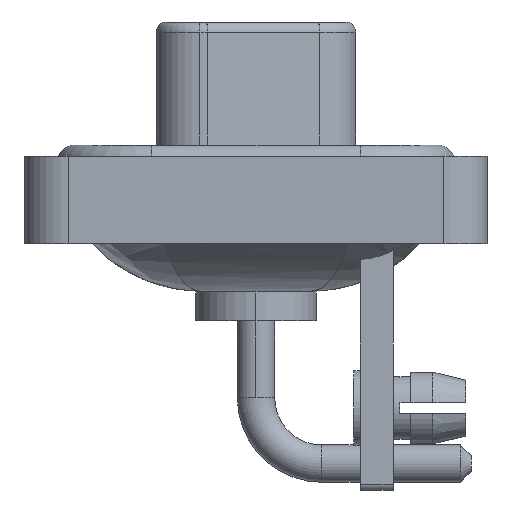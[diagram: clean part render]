
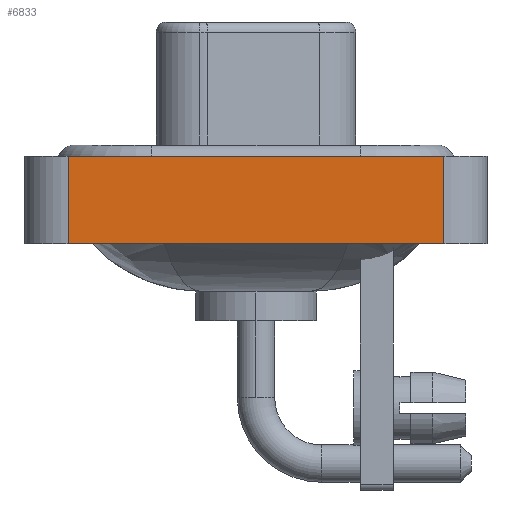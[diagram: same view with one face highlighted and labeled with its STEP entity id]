
A CAD part, left-side view. The second image highlights one B-rep face of the part: STEP entity #6833.
In plain terms, the highlighted planar face has unit normal (-1, 0, 0).
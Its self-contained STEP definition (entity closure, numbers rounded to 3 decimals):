
#43 = CARTESIAN_POINT ( 'NONE',  ( -7.35, -8.55, -3.6 ) ) ;
#666 = CARTESIAN_POINT ( 'NONE',  ( -7.35, 8.55, -3.6 ) ) ;
#1104 = DIRECTION ( 'NONE',  ( 0., 0., 1. ) ) ;
#1504 = VERTEX_POINT ( 'NONE', #3130 ) ;
#1951 = ORIENTED_EDGE ( 'NONE', *, *, #7574, .T. ) ;
#2190 = DIRECTION ( 'NONE',  ( 0., -1., 0. ) ) ;
#3130 = CARTESIAN_POINT ( 'NONE',  ( -7.35, 8.55, -3.6 ) ) ;
#3673 = DIRECTION ( 'NONE',  ( 0., 0., 1. ) ) ;
#3852 = CARTESIAN_POINT ( 'NONE',  ( -7.35, 8.55, 0.4 ) ) ;
#4061 = VECTOR ( 'NONE', #9887, 1000. ) ;
#4066 = VERTEX_POINT ( 'NONE', #43 ) ;
#4511 = CARTESIAN_POINT ( 'NONE',  ( -7.35, -8.55, -3.6 ) ) ;
#5186 = LINE ( 'NONE', #8392, #17404 ) ;
#5952 = FACE_OUTER_BOUND ( 'NONE', #19477, .T. ) ;
#5972 = EDGE_CURVE ( 'NONE', #4066, #20293, #17813, .T. ) ;
#6833 = ADVANCED_FACE ( 'NONE', ( #5952 ), #15697, .T. ) ;
#7574 = EDGE_CURVE ( 'NONE', #1504, #4066, #5186, .T. ) ;
#8015 = LINE ( 'NONE', #14460, #4061 ) ;
#8392 = CARTESIAN_POINT ( 'NONE',  ( -7.35, -8.55, -3.6 ) ) ;
#9370 = CARTESIAN_POINT ( 'NONE',  ( -7.35, -8.55, 0.4 ) ) ;
#9724 = AXIS2_PLACEMENT_3D ( 'NONE', #4511, #10626, #1104 ) ;
#9887 = DIRECTION ( 'NONE',  ( 0., -1., 0. ) ) ;
#9923 = CARTESIAN_POINT ( 'NONE',  ( -7.35, -8.55, -3.6 ) ) ;
#10433 = ORIENTED_EDGE ( 'NONE', *, *, #12116, .F. ) ;
#10626 = DIRECTION ( 'NONE',  ( -1., 0., 0. ) ) ;
#10729 = VECTOR ( 'NONE', #16255, 1000. ) ;
#12116 = EDGE_CURVE ( 'NONE', #17811, #20293, #8015, .T. ) ;
#13508 = VECTOR ( 'NONE', #3673, 1000. ) ;
#13545 = EDGE_CURVE ( 'NONE', #1504, #17811, #17882, .T. ) ;
#14460 = CARTESIAN_POINT ( 'NONE',  ( -7.35, -8.55, 0.4 ) ) ;
#15697 = PLANE ( 'NONE',  #9724 ) ;
#16255 = DIRECTION ( 'NONE',  ( 0., 0., 1. ) ) ;
#16682 = ORIENTED_EDGE ( 'NONE', *, *, #13545, .F. ) ;
#17404 = VECTOR ( 'NONE', #2190, 1000. ) ;
#17811 = VERTEX_POINT ( 'NONE', #3852 ) ;
#17813 = LINE ( 'NONE', #9923, #10729 ) ;
#17882 = LINE ( 'NONE', #666, #13508 ) ;
#18726 = ORIENTED_EDGE ( 'NONE', *, *, #5972, .T. ) ;
#19477 = EDGE_LOOP ( 'NONE', ( #18726, #10433, #16682, #1951 ) ) ;
#20293 = VERTEX_POINT ( 'NONE', #9370 ) ;
